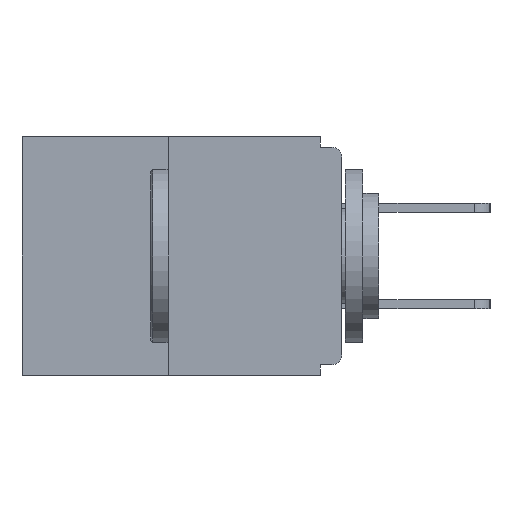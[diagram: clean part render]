
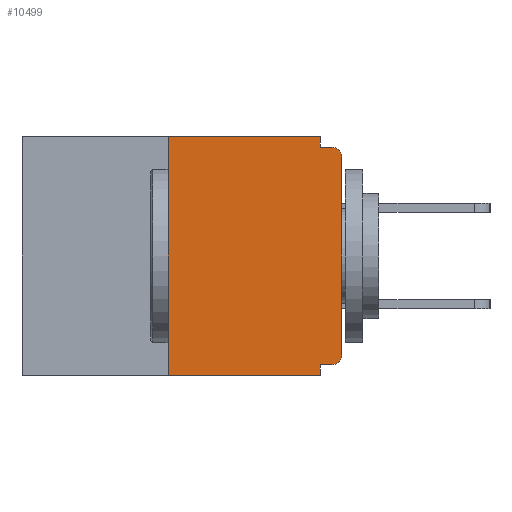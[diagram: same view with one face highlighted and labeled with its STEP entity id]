
A CAD part, left-side view. The second image highlights one B-rep face of the part: STEP entity #10499.
In plain terms, the highlighted planar face has unit normal (-1, 0, 0).
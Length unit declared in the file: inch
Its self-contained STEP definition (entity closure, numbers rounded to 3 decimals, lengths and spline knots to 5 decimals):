
#738 = CARTESIAN_POINT ( 'NONE',  ( 0., 0.031, -0.328 ) ) ;
#829 = ORIENTED_EDGE ( 'NONE', *, *, #11836, .T. ) ;
#945 = EDGE_CURVE ( 'NONE', #10955, #3731, #8833, .T. ) ;
#1017 = CARTESIAN_POINT ( 'NONE',  ( 0., 0.25, 0. ) ) ;
#1096 = EDGE_CURVE ( 'NONE', #8459, #11655, #12259, .T. ) ;
#1187 = LINE ( 'NONE', #2960, #13470 ) ;
#1889 = CARTESIAN_POINT ( 'NONE',  ( 0., 0.031, 0. ) ) ;
#2018 = AXIS2_PLACEMENT_3D ( 'NONE', #2345, #9708, #3278 ) ;
#2310 = EDGE_CURVE ( 'NONE', #3785, #10433, #7600, .T. ) ;
#2345 = CARTESIAN_POINT ( 'NONE',  ( 0., 0.015, -0.313 ) ) ;
#2721 = DIRECTION ( 'NONE',  ( 0., -1., 0. ) ) ;
#2811 = CARTESIAN_POINT ( 'NONE',  ( 0., 0., 0. ) ) ;
#2960 = CARTESIAN_POINT ( 'NONE',  ( 0., 0.46, 0. ) ) ;
#2962 = ORIENTED_EDGE ( 'NONE', *, *, #5078, .F. ) ;
#3238 = CARTESIAN_POINT ( 'NONE',  ( 0., 0.015, -0.328 ) ) ;
#3270 = ORIENTED_EDGE ( 'NONE', *, *, #6615, .F. ) ;
#3278 = DIRECTION ( 'NONE',  ( 0., 0., -1. ) ) ;
#3731 = VERTEX_POINT ( 'NONE', #5074 ) ;
#3785 = VERTEX_POINT ( 'NONE', #12437 ) ;
#3841 = DIRECTION ( 'NONE',  ( 0., -1., 0. ) ) ;
#3860 = CARTESIAN_POINT ( 'NONE',  ( 0., 0., -0.313 ) ) ;
#3955 = DIRECTION ( 'NONE',  ( 0., 0., -1. ) ) ;
#4012 = EDGE_LOOP ( 'NONE', ( #2962, #8047, #4181, #7796, #6883, #829, #12712, #10977, #3270, #8522 ) ) ;
#4181 = ORIENTED_EDGE ( 'NONE', *, *, #945, .T. ) ;
#4379 = CARTESIAN_POINT ( 'NONE',  ( 0., 0.015, -0.015 ) ) ;
#4670 = LINE ( 'NONE', #2811, #9691 ) ;
#4735 = CARTESIAN_POINT ( 'NONE',  ( 0., 0.031, -0.343 ) ) ;
#4810 = DIRECTION ( 'NONE',  ( 0., 0., -1. ) ) ;
#4823 = VECTOR ( 'NONE', #4810, 39.37008 ) ;
#5074 = CARTESIAN_POINT ( 'NONE',  ( 0., 0.031, -0.343 ) ) ;
#5078 = EDGE_CURVE ( 'NONE', #7712, #8459, #1187, .T. ) ;
#5462 = EDGE_CURVE ( 'NONE', #5966, #3731, #6157, .T. ) ;
#5542 = EDGE_CURVE ( 'NONE', #8240, #3785, #4670, .T. ) ;
#5764 = DIRECTION ( 'NONE',  ( 0., 0., -1. ) ) ;
#5813 = AXIS2_PLACEMENT_3D ( 'NONE', #6464, #13502, #5764 ) ;
#5966 = VERTEX_POINT ( 'NONE', #738 ) ;
#6157 = LINE ( 'NONE', #4735, #4823 ) ;
#6337 = CARTESIAN_POINT ( 'NONE',  ( 0., 0., -0.328 ) ) ;
#6353 = DIRECTION ( 'NONE',  ( 0., 0., -1. ) ) ;
#6464 = CARTESIAN_POINT ( 'NONE',  ( 0., 0.46, 0. ) ) ;
#6615 = EDGE_CURVE ( 'NONE', #11655, #10433, #11247, .T. ) ;
#6808 = EDGE_CURVE ( 'NONE', #6852, #5966, #12740, .T. ) ;
#6852 = VERTEX_POINT ( 'NONE', #3238 ) ;
#6883 = ORIENTED_EDGE ( 'NONE', *, *, #6808, .F. ) ;
#7038 = DIRECTION ( 'NONE',  ( 0., 0., 1. ) ) ;
#7600 = CIRCLE ( 'NONE', #13479, 0.015 ) ;
#7712 = VERTEX_POINT ( 'NONE', #1017 ) ;
#7762 = DIRECTION ( 'NONE',  ( 0., 0., 1. ) ) ;
#7796 = ORIENTED_EDGE ( 'NONE', *, *, #5462, .F. ) ;
#8047 = ORIENTED_EDGE ( 'NONE', *, *, #8082, .F. ) ;
#8082 = EDGE_CURVE ( 'NONE', #10955, #7712, #12504, .T. ) ;
#8240 = VERTEX_POINT ( 'NONE', #3860 ) ;
#8433 = PLANE ( 'NONE',  #5813 ) ;
#8459 = VERTEX_POINT ( 'NONE', #10554 ) ;
#8472 = CIRCLE ( 'NONE', #2018, 0.015 ) ;
#8522 = ORIENTED_EDGE ( 'NONE', *, *, #1096, .F. ) ;
#8531 = CARTESIAN_POINT ( 'NONE',  ( 0., 0.031, -0.015 ) ) ;
#8833 = LINE ( 'NONE', #10266, #12781 ) ;
#8907 = CARTESIAN_POINT ( 'NONE',  ( 0., 0.25, 0. ) ) ;
#9535 = DIRECTION ( 'NONE',  ( -1., 0., 0. ) ) ;
#9691 = VECTOR ( 'NONE', #7038, 39.37008 ) ;
#9708 = DIRECTION ( 'NONE',  ( -1., 0., 0. ) ) ;
#10214 = CARTESIAN_POINT ( 'NONE',  ( 0., 0., -0.015 ) ) ;
#10266 = CARTESIAN_POINT ( 'NONE',  ( 0., 0.46, -0.343 ) ) ;
#10411 = DIRECTION ( 'NONE',  ( 0., -1., 0. ) ) ;
#10433 = VERTEX_POINT ( 'NONE', #4379 ) ;
#10499 = ADVANCED_FACE ( 'NONE', ( #11317 ), #8433, .F. ) ;
#10554 = CARTESIAN_POINT ( 'NONE',  ( 0., 0.031, 0. ) ) ;
#10630 = DIRECTION ( 'NONE',  ( 0., 1., 0. ) ) ;
#10763 = VECTOR ( 'NONE', #3841, 39.37008 ) ;
#10955 = VERTEX_POINT ( 'NONE', #12404 ) ;
#10977 = ORIENTED_EDGE ( 'NONE', *, *, #2310, .T. ) ;
#11247 = LINE ( 'NONE', #10214, #10763 ) ;
#11317 = FACE_OUTER_BOUND ( 'NONE', #4012, .T. ) ;
#11616 = VECTOR ( 'NONE', #3955, 39.37008 ) ;
#11655 = VERTEX_POINT ( 'NONE', #8531 ) ;
#11836 = EDGE_CURVE ( 'NONE', #6852, #8240, #8472, .T. ) ;
#12065 = VECTOR ( 'NONE', #10630, 39.37008 ) ;
#12259 = LINE ( 'NONE', #1889, #11616 ) ;
#12404 = CARTESIAN_POINT ( 'NONE',  ( 0., 0.25, -0.343 ) ) ;
#12437 = CARTESIAN_POINT ( 'NONE',  ( 0., 0., -0.03 ) ) ;
#12504 = LINE ( 'NONE', #8907, #12697 ) ;
#12697 = VECTOR ( 'NONE', #7762, 39.37008 ) ;
#12712 = ORIENTED_EDGE ( 'NONE', *, *, #5542, .T. ) ;
#12740 = LINE ( 'NONE', #6337, #12065 ) ;
#12781 = VECTOR ( 'NONE', #2721, 39.37008 ) ;
#13470 = VECTOR ( 'NONE', #10411, 39.37008 ) ;
#13479 = AXIS2_PLACEMENT_3D ( 'NONE', #13678, #9535, #6353 ) ;
#13502 = DIRECTION ( 'NONE',  ( 1., 0., 0. ) ) ;
#13678 = CARTESIAN_POINT ( 'NONE',  ( 0., 0.015, -0.03 ) ) ;
